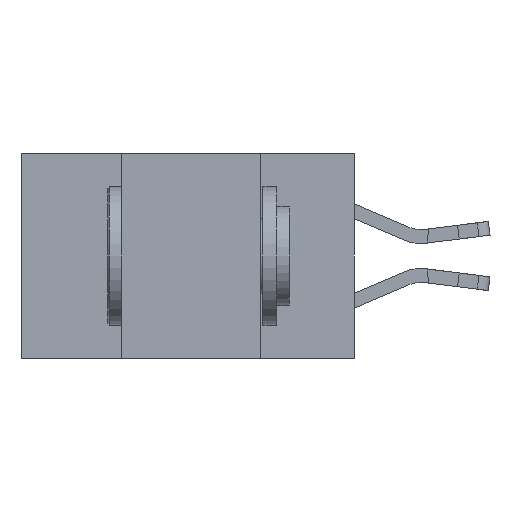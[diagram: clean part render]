
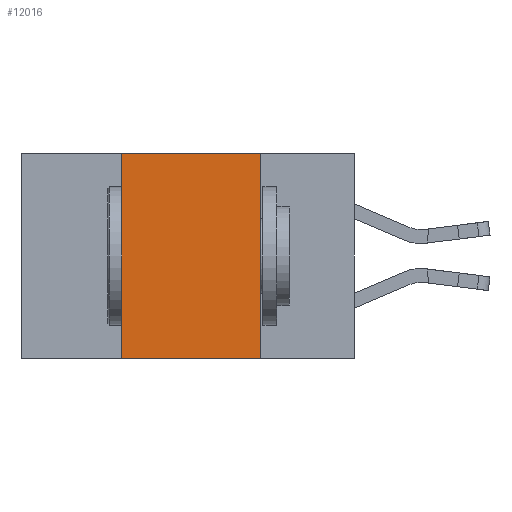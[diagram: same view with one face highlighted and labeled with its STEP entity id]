
A CAD part, left-side view. The second image highlights one B-rep face of the part: STEP entity #12016.
In plain terms, the highlighted planar face has unit normal (-1, 0, 0).
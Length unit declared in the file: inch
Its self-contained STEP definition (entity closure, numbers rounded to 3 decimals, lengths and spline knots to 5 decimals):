
#132 = VERTEX_POINT ( 'NONE', #1021 ) ;
#221 = VERTEX_POINT ( 'NONE', #9497 ) ;
#553 = EDGE_CURVE ( 'NONE', #221, #15625, #15043, .T. ) ;
#1021 = CARTESIAN_POINT ( 'NONE',  ( 0., 0.42, 0. ) ) ;
#1278 = VECTOR ( 'NONE', #5831, 39.37008 ) ;
#1641 = CARTESIAN_POINT ( 'NONE',  ( 0., 0.17, -0.37 ) ) ;
#2300 = EDGE_CURVE ( 'NONE', #132, #5724, #15129, .T. ) ;
#2481 = DIRECTION ( 'NONE',  ( 0., -1., 0. ) ) ;
#2553 = CARTESIAN_POINT ( 'NONE',  ( 0., 0.42, -0.37 ) ) ;
#2837 = DIRECTION ( 'NONE',  ( 1., 0., 0. ) ) ;
#3013 = CARTESIAN_POINT ( 'NONE',  ( 0., 0.17, 0. ) ) ;
#3846 = CARTESIAN_POINT ( 'NONE',  ( 0., 0.6, 0. ) ) ;
#3908 = VECTOR ( 'NONE', #13642, 39.37008 ) ;
#4424 = PLANE ( 'NONE',  #6703 ) ;
#4970 = VECTOR ( 'NONE', #2481, 39.37008 ) ;
#5653 = CARTESIAN_POINT ( 'NONE',  ( 0., 0.6, -0.37 ) ) ;
#5724 = VERTEX_POINT ( 'NONE', #3013 ) ;
#5831 = DIRECTION ( 'NONE',  ( 0., 0., 1. ) ) ;
#6014 = DIRECTION ( 'NONE',  ( 0., 0., -1. ) ) ;
#6703 = AXIS2_PLACEMENT_3D ( 'NONE', #11023, #2837, #6014 ) ;
#7393 = EDGE_LOOP ( 'NONE', ( #14427, #20508, #16631, #7727 ) ) ;
#7727 = ORIENTED_EDGE ( 'NONE', *, *, #553, .T. ) ;
#9497 = CARTESIAN_POINT ( 'NONE',  ( 0., 0.42, -0.37 ) ) ;
#9801 = VECTOR ( 'NONE', #10763, 39.37008 ) ;
#10763 = DIRECTION ( 'NONE',  ( 0., 0., -1. ) ) ;
#11023 = CARTESIAN_POINT ( 'NONE',  ( 0., 0.6, 0. ) ) ;
#11474 = EDGE_CURVE ( 'NONE', #221, #132, #15622, .T. ) ;
#12016 = ADVANCED_FACE ( 'NONE', ( #20581 ), #4424, .F. ) ;
#12862 = EDGE_CURVE ( 'NONE', #5724, #15625, #18834, .T. ) ;
#13642 = DIRECTION ( 'NONE',  ( 0., -1., 0. ) ) ;
#14427 = ORIENTED_EDGE ( 'NONE', *, *, #12862, .F. ) ;
#15043 = LINE ( 'NONE', #5653, #4970 ) ;
#15129 = LINE ( 'NONE', #3846, #3908 ) ;
#15622 = LINE ( 'NONE', #2553, #1278 ) ;
#15625 = VERTEX_POINT ( 'NONE', #1641 ) ;
#15965 = CARTESIAN_POINT ( 'NONE',  ( 0., 0.17, -0.37 ) ) ;
#16631 = ORIENTED_EDGE ( 'NONE', *, *, #11474, .F. ) ;
#18834 = LINE ( 'NONE', #15965, #9801 ) ;
#20508 = ORIENTED_EDGE ( 'NONE', *, *, #2300, .F. ) ;
#20581 = FACE_OUTER_BOUND ( 'NONE', #7393, .T. ) ;
